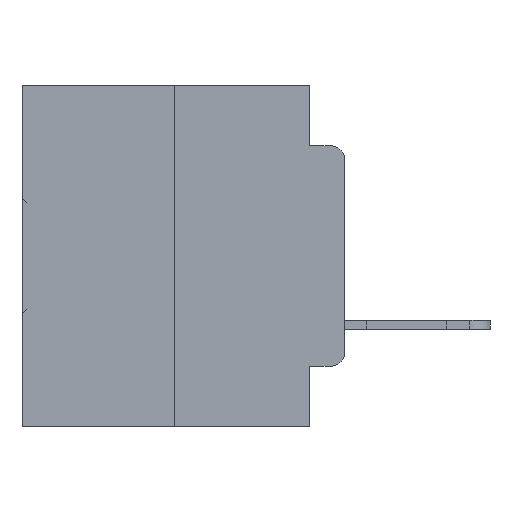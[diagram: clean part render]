
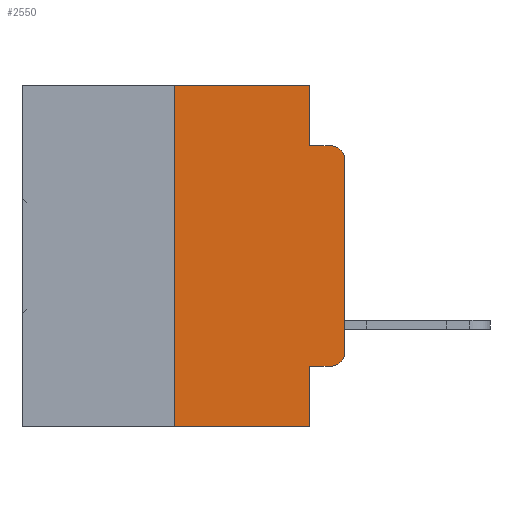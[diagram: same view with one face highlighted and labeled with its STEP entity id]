
A CAD part, left-side view. The second image highlights one B-rep face of the part: STEP entity #2550.
In plain terms, the highlighted planar face has unit normal (-1, 0, 0).
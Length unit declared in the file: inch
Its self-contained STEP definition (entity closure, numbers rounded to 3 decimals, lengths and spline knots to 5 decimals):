
#710 = VERTEX_POINT ( 'NONE', #20687 ) ;
#778 = LINE ( 'NONE', #20892, #6618 ) ;
#789 = CARTESIAN_POINT ( 'NONE',  ( 0., 0.051, 0. ) ) ;
#1373 = VERTEX_POINT ( 'NONE', #12214 ) ;
#1602 = CARTESIAN_POINT ( 'NONE',  ( 0., 0.25, 0. ) ) ;
#1690 = EDGE_CURVE ( 'NONE', #1373, #710, #5673, .T. ) ;
#1969 = VECTOR ( 'NONE', #2531, 39.37008 ) ;
#2155 = CARTESIAN_POINT ( 'NONE',  ( 0., 0.02, -0.4115 ) ) ;
#2531 = DIRECTION ( 'NONE',  ( 0., -1., 0. ) ) ;
#2550 = ADVANCED_FACE ( 'NONE', ( #26055 ), #24981, .F. ) ;
#2587 = ORIENTED_EDGE ( 'NONE', *, *, #15114, .T. ) ;
#2707 = CARTESIAN_POINT ( 'NONE',  ( 0., 0.473, 0. ) ) ;
#2848 = DIRECTION ( 'NONE',  ( 0., 0., -1. ) ) ;
#3267 = DIRECTION ( 'NONE',  ( -1., 0., 0. ) ) ;
#3281 = VECTOR ( 'NONE', #17026, 39.37008 ) ;
#3420 = CARTESIAN_POINT ( 'NONE',  ( 0., 0.02, -0.1085 ) ) ;
#4148 = VERTEX_POINT ( 'NONE', #20019 ) ;
#4175 = ORIENTED_EDGE ( 'NONE', *, *, #5570, .T. ) ;
#5289 = LINE ( 'NONE', #15879, #25056 ) ;
#5570 = EDGE_CURVE ( 'NONE', #21057, #1373, #23000, .T. ) ;
#5621 = EDGE_CURVE ( 'NONE', #26545, #29195, #7760, .T. ) ;
#5673 = CIRCLE ( 'NONE', #21527, 0.02 ) ;
#6618 = VECTOR ( 'NONE', #13276, 39.37008 ) ;
#6906 = CARTESIAN_POINT ( 'NONE',  ( 0., 0.02, -0.3915 ) ) ;
#7292 = CIRCLE ( 'NONE', #28626, 0.02 ) ;
#7760 = LINE ( 'NONE', #2707, #13085 ) ;
#7965 = DIRECTION ( 'NONE',  ( 0., -1., 0. ) ) ;
#8866 = ORIENTED_EDGE ( 'NONE', *, *, #31636, .F. ) ;
#8946 = ORIENTED_EDGE ( 'NONE', *, *, #1690, .T. ) ;
#9278 = VECTOR ( 'NONE', #15154, 39.37008 ) ;
#9660 = DIRECTION ( 'NONE',  ( 0., 0., -1. ) ) ;
#9733 = CARTESIAN_POINT ( 'NONE',  ( 0., 0.25, -0.5 ) ) ;
#11148 = ORIENTED_EDGE ( 'NONE', *, *, #23515, .F. ) ;
#11559 = CARTESIAN_POINT ( 'NONE',  ( 0., 0., -0.3915 ) ) ;
#11789 = ORIENTED_EDGE ( 'NONE', *, *, #18540, .T. ) ;
#12212 = ORIENTED_EDGE ( 'NONE', *, *, #25218, .F. ) ;
#12214 = CARTESIAN_POINT ( 'NONE',  ( 0., 0., -0.1085 ) ) ;
#13085 = VECTOR ( 'NONE', #21191, 39.37008 ) ;
#13229 = CARTESIAN_POINT ( 'NONE',  ( 0., 0.051, 0. ) ) ;
#13276 = DIRECTION ( 'NONE',  ( 0., 0., -1. ) ) ;
#14731 = EDGE_LOOP ( 'NONE', ( #4175, #8946, #8866, #33240, #14874, #12212, #17608, #11148, #11789, #2587 ) ) ;
#14806 = VERTEX_POINT ( 'NONE', #24915 ) ;
#14874 = ORIENTED_EDGE ( 'NONE', *, *, #5621, .F. ) ;
#15114 = EDGE_CURVE ( 'NONE', #25937, #21057, #7292, .T. ) ;
#15154 = DIRECTION ( 'NONE',  ( 0., 0., 1. ) ) ;
#15781 = CARTESIAN_POINT ( 'NONE',  ( 0., 0., 0. ) ) ;
#15879 = CARTESIAN_POINT ( 'NONE',  ( 0., 0.473, -0.5 ) ) ;
#16193 = LINE ( 'NONE', #1602, #9278 ) ;
#17026 = DIRECTION ( 'NONE',  ( 0., 0., -1. ) ) ;
#17608 = ORIENTED_EDGE ( 'NONE', *, *, #27686, .T. ) ;
#17736 = CARTESIAN_POINT ( 'NONE',  ( 0., 0.25, 0. ) ) ;
#17934 = VERTEX_POINT ( 'NONE', #9733 ) ;
#18540 = EDGE_CURVE ( 'NONE', #14806, #25937, #31121, .T. ) ;
#20019 = CARTESIAN_POINT ( 'NONE',  ( 0., 0.051, -0.0885 ) ) ;
#20687 = CARTESIAN_POINT ( 'NONE',  ( 0., 0.02, -0.0885 ) ) ;
#20775 = CARTESIAN_POINT ( 'NONE',  ( 0., 0.051, -0.4115 ) ) ;
#20892 = CARTESIAN_POINT ( 'NONE',  ( 0., 0.051, 0. ) ) ;
#21057 = VERTEX_POINT ( 'NONE', #11559 ) ;
#21191 = DIRECTION ( 'NONE',  ( 0., -1., 0. ) ) ;
#21527 = AXIS2_PLACEMENT_3D ( 'NONE', #3420, #3267, #2848 ) ;
#23000 = LINE ( 'NONE', #15781, #30254 ) ;
#23266 = VERTEX_POINT ( 'NONE', #30889 ) ;
#23498 = CARTESIAN_POINT ( 'NONE',  ( 0., 0.051, -0.0885 ) ) ;
#23515 = EDGE_CURVE ( 'NONE', #14806, #23266, #24066, .T. ) ;
#24066 = LINE ( 'NONE', #789, #3281 ) ;
#24642 = DIRECTION ( 'NONE',  ( 0., 0., -1. ) ) ;
#24692 = DIRECTION ( 'NONE',  ( 1., 0., 0. ) ) ;
#24882 = DIRECTION ( 'NONE',  ( -1., 0., 0. ) ) ;
#24915 = CARTESIAN_POINT ( 'NONE',  ( 0., 0.051, -0.4115 ) ) ;
#24981 = PLANE ( 'NONE',  #31929 ) ;
#25056 = VECTOR ( 'NONE', #7965, 39.37008 ) ;
#25218 = EDGE_CURVE ( 'NONE', #17934, #26545, #16193, .T. ) ;
#25937 = VERTEX_POINT ( 'NONE', #2155 ) ;
#26055 = FACE_OUTER_BOUND ( 'NONE', #14731, .T. ) ;
#26138 = CARTESIAN_POINT ( 'NONE',  ( 0., 0.473, 0. ) ) ;
#26545 = VERTEX_POINT ( 'NONE', #17736 ) ;
#26819 = EDGE_CURVE ( 'NONE', #29195, #4148, #778, .T. ) ;
#27686 = EDGE_CURVE ( 'NONE', #17934, #23266, #5289, .T. ) ;
#28626 = AXIS2_PLACEMENT_3D ( 'NONE', #6906, #24882, #9660 ) ;
#29195 = VERTEX_POINT ( 'NONE', #13229 ) ;
#29655 = VECTOR ( 'NONE', #32932, 39.37008 ) ;
#30222 = LINE ( 'NONE', #23498, #1969 ) ;
#30254 = VECTOR ( 'NONE', #32926, 39.37008 ) ;
#30889 = CARTESIAN_POINT ( 'NONE',  ( 0., 0.051, -0.5 ) ) ;
#31121 = LINE ( 'NONE', #20775, #29655 ) ;
#31636 = EDGE_CURVE ( 'NONE', #4148, #710, #30222, .T. ) ;
#31929 = AXIS2_PLACEMENT_3D ( 'NONE', #26138, #24692, #24642 ) ;
#32926 = DIRECTION ( 'NONE',  ( 0., 0., 1. ) ) ;
#32932 = DIRECTION ( 'NONE',  ( 0., -1., 0. ) ) ;
#33240 = ORIENTED_EDGE ( 'NONE', *, *, #26819, .F. ) ;
